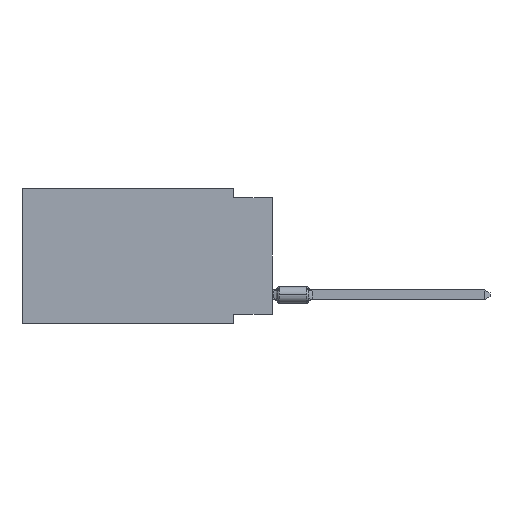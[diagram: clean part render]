
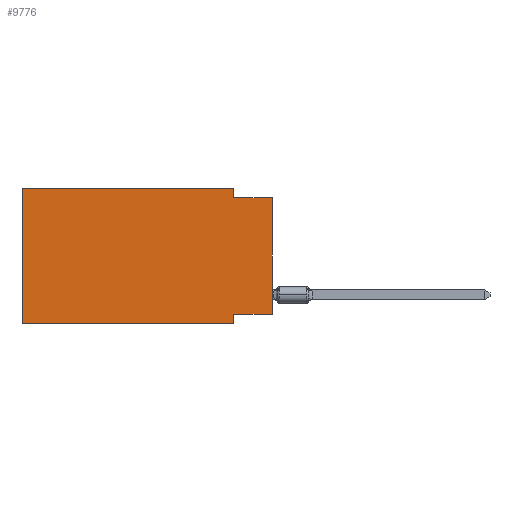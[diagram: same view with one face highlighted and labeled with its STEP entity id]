
A CAD part, left-side view. The second image highlights one B-rep face of the part: STEP entity #9776.
In plain terms, the highlighted planar face has unit normal (-1, 0, 0).
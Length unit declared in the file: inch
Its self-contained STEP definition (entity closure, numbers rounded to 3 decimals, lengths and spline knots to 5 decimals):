
#90 = EDGE_CURVE ( 'NONE', #4941, #7796, #16759, .T. ) ;
#107 = VECTOR ( 'NONE', #4904, 39.37008 ) ;
#126 = VECTOR ( 'NONE', #2467, 39.37008 ) ;
#185 = CARTESIAN_POINT ( 'NONE',  ( 0., 0., -0.325 ) ) ;
#827 = LINE ( 'NONE', #14463, #884 ) ;
#884 = VECTOR ( 'NONE', #6304, 39.37008 ) ;
#1262 = DIRECTION ( 'NONE',  ( 0., 0., -1. ) ) ;
#1326 = ORIENTED_EDGE ( 'NONE', *, *, #14127, .F. ) ;
#1967 = LINE ( 'NONE', #15525, #15325 ) ;
#2085 = PLANE ( 'NONE',  #7586 ) ;
#2209 = VERTEX_POINT ( 'NONE', #15696 ) ;
#2467 = DIRECTION ( 'NONE',  ( 0., -1., 0. ) ) ;
#2929 = CARTESIAN_POINT ( 'NONE',  ( 0., 0.645, 0. ) ) ;
#4001 = CARTESIAN_POINT ( 'NONE',  ( 0., 0.645, -0.35 ) ) ;
#4085 = LINE ( 'NONE', #13800, #10082 ) ;
#4172 = VERTEX_POINT ( 'NONE', #6599 ) ;
#4682 = VERTEX_POINT ( 'NONE', #7201 ) ;
#4904 = DIRECTION ( 'NONE',  ( 0., 0., -1. ) ) ;
#4941 = VERTEX_POINT ( 'NONE', #4001 ) ;
#5003 = CARTESIAN_POINT ( 'NONE',  ( 0., 0.645, 0. ) ) ;
#5159 = ORIENTED_EDGE ( 'NONE', *, *, #17105, .F. ) ;
#6274 = LINE ( 'NONE', #16170, #107 ) ;
#6304 = DIRECTION ( 'NONE',  ( 0., 1., 0. ) ) ;
#6599 = CARTESIAN_POINT ( 'NONE',  ( 0., 0., -0.025 ) ) ;
#6752 = LINE ( 'NONE', #15013, #126 ) ;
#7201 = CARTESIAN_POINT ( 'NONE',  ( 0., 0.1, -0.35 ) ) ;
#7586 = AXIS2_PLACEMENT_3D ( 'NONE', #5003, #14721, #10588 ) ;
#7796 = VERTEX_POINT ( 'NONE', #15953 ) ;
#7936 = CARTESIAN_POINT ( 'NONE',  ( 0., 0.1, -0.325 ) ) ;
#7998 = ORIENTED_EDGE ( 'NONE', *, *, #12589, .T. ) ;
#8133 = CARTESIAN_POINT ( 'NONE',  ( 0., 0.1, 0. ) ) ;
#8163 = EDGE_CURVE ( 'NONE', #14334, #14585, #827, .T. ) ;
#8240 = VERTEX_POINT ( 'NONE', #8133 ) ;
#8345 = VECTOR ( 'NONE', #12809, 39.37008 ) ;
#8347 = ORIENTED_EDGE ( 'NONE', *, *, #16504, .F. ) ;
#9124 = LINE ( 'NONE', #12138, #11523 ) ;
#9776 = ADVANCED_FACE ( 'NONE', ( #17560 ), #2085, .F. ) ;
#10082 = VECTOR ( 'NONE', #1262, 39.37008 ) ;
#10293 = VECTOR ( 'NONE', #12057, 39.37008 ) ;
#10588 = DIRECTION ( 'NONE',  ( 0., 0., -1. ) ) ;
#10596 = LINE ( 'NONE', #14639, #10293 ) ;
#11523 = VECTOR ( 'NONE', #17738, 39.37008 ) ;
#11556 = EDGE_LOOP ( 'NONE', ( #7998, #5159, #1326, #8347, #14535, #16912, #13782, #15224 ) ) ;
#12057 = DIRECTION ( 'NONE',  ( 0., 0., 1. ) ) ;
#12138 = CARTESIAN_POINT ( 'NONE',  ( 0., 0.645, -0.35 ) ) ;
#12589 = EDGE_CURVE ( 'NONE', #14334, #4172, #10596, .T. ) ;
#12809 = DIRECTION ( 'NONE',  ( 0., 0., 1. ) ) ;
#13782 = ORIENTED_EDGE ( 'NONE', *, *, #17707, .F. ) ;
#13800 = CARTESIAN_POINT ( 'NONE',  ( 0., 0.1, -0.35 ) ) ;
#14127 = EDGE_CURVE ( 'NONE', #8240, #2209, #6274, .T. ) ;
#14334 = VERTEX_POINT ( 'NONE', #185 ) ;
#14463 = CARTESIAN_POINT ( 'NONE',  ( 0., 0., -0.325 ) ) ;
#14535 = ORIENTED_EDGE ( 'NONE', *, *, #90, .F. ) ;
#14585 = VERTEX_POINT ( 'NONE', #7936 ) ;
#14639 = CARTESIAN_POINT ( 'NONE',  ( 0., 0., 0. ) ) ;
#14721 = DIRECTION ( 'NONE',  ( 1., 0., 0. ) ) ;
#15013 = CARTESIAN_POINT ( 'NONE',  ( 0., 0., -0.025 ) ) ;
#15224 = ORIENTED_EDGE ( 'NONE', *, *, #8163, .F. ) ;
#15325 = VECTOR ( 'NONE', #15879, 39.37008 ) ;
#15525 = CARTESIAN_POINT ( 'NONE',  ( 0., 0.645, 0. ) ) ;
#15696 = CARTESIAN_POINT ( 'NONE',  ( 0., 0.1, -0.025 ) ) ;
#15879 = DIRECTION ( 'NONE',  ( 0., -1., 0. ) ) ;
#15953 = CARTESIAN_POINT ( 'NONE',  ( 0., 0.645, 0. ) ) ;
#16170 = CARTESIAN_POINT ( 'NONE',  ( 0., 0.1, 0. ) ) ;
#16504 = EDGE_CURVE ( 'NONE', #7796, #8240, #1967, .T. ) ;
#16759 = LINE ( 'NONE', #2929, #8345 ) ;
#16912 = ORIENTED_EDGE ( 'NONE', *, *, #17553, .T. ) ;
#17105 = EDGE_CURVE ( 'NONE', #2209, #4172, #6752, .T. ) ;
#17553 = EDGE_CURVE ( 'NONE', #4941, #4682, #9124, .T. ) ;
#17560 = FACE_OUTER_BOUND ( 'NONE', #11556, .T. ) ;
#17707 = EDGE_CURVE ( 'NONE', #14585, #4682, #4085, .T. ) ;
#17738 = DIRECTION ( 'NONE',  ( 0., -1., 0. ) ) ;
